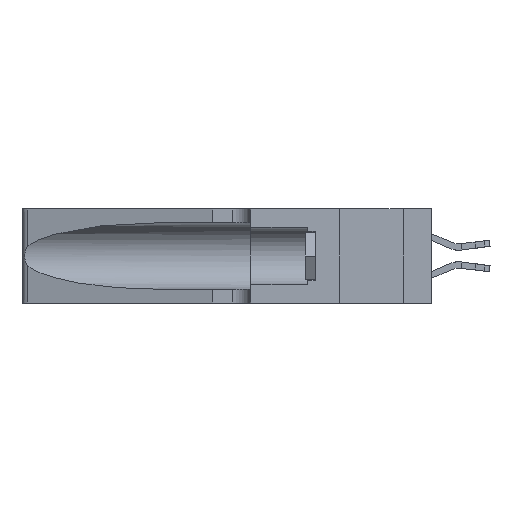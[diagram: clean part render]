
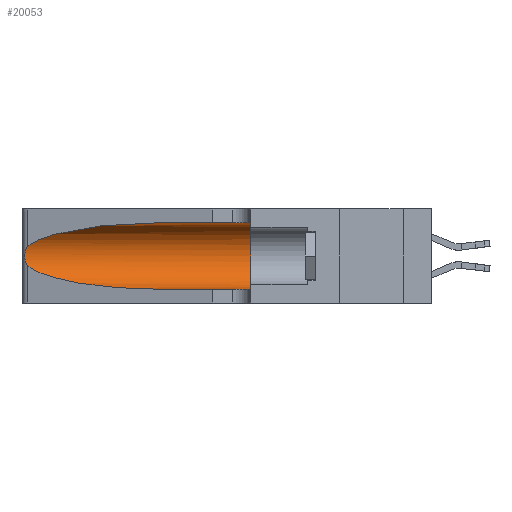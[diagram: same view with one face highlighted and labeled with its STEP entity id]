
A CAD part, left-side view. The second image highlights one B-rep face of the part: STEP entity #20053.
In plain terms, the highlighted cylindrical face has radius 3.308 mm (diameter 6.617 mm), a partial arc.
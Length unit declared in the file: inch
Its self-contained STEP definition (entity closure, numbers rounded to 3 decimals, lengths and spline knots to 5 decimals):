
#73 = B_SPLINE_CURVE_WITH_KNOTS ( 'NONE', 3,
 ( #13651, #1117, #9318, #3295, #23858, #24483, #26565, #3387, #9953, #1459, #24572, #22647, #10691, #15704 ),
 .UNSPECIFIED., .F., .F.,
 ( 4, 2, 2, 2, 2, 2, 4 ),
 ( 0., 0.00027, 0.00053, 0.00107, 0.0016, 0.00187, 0.00214 ),
 .UNSPECIFIED. ) ;
#98 = DIRECTION ( 'NONE',  ( 0., -1., 0. ) ) ;
#560 = ORIENTED_EDGE ( 'NONE', *, *, #17639, .T. ) ;
#666 = VERTEX_POINT ( 'NONE', #25088 ) ;
#972 = DIRECTION ( 'NONE',  ( 0., -1., 0. ) ) ;
#1107 = DIRECTION ( 'NONE',  ( 0., 0., 1. ) ) ;
#1117 = CARTESIAN_POINT ( 'NONE',  ( 0.25555, 1.22994, 0.2215 ) ) ;
#1459 = CARTESIAN_POINT ( 'NONE',  ( 0.25856, 1.23593, 0.16098 ) ) ;
#1947 = CARTESIAN_POINT ( 'NONE',  ( 0.2373, 1.15595, 0.08982 ) ) ;
#2285 = VERTEX_POINT ( 'NONE', #23830 ) ;
#2407 =( BOUNDED_CURVE ( )  B_SPLINE_CURVE ( 3, ( #6044, #1947, #22855, #18428 ),
 .UNSPECIFIED., .F., .F. ) 
 B_SPLINE_CURVE_WITH_KNOTS ( ( 4, 4 ),
 ( 3.44316, 4.71239 ),
 .UNSPECIFIED. ) 
 CURVE ( )  GEOMETRIC_REPRESENTATION_ITEM ( )  RATIONAL_B_SPLINE_CURVE ( ( 1., 0.87, 0.87, 1. ) ) 
 REPRESENTATION_ITEM ( '' )  );
#2459 = VECTOR ( 'NONE', #98, 39.37008 ) ;
#2837 = LINE ( 'NONE', #11319, #24513 ) ;
#3295 = CARTESIAN_POINT ( 'NONE',  ( 0.25787, 1.23484, 0.2124 ) ) ;
#3387 = CARTESIAN_POINT ( 'NONE',  ( 0.26075, 1.23896, 0.178 ) ) ;
#4401 =( BOUNDED_CURVE ( )  B_SPLINE_CURVE ( 3, ( #18512, #8134, #5947, #8233 ),
 .UNSPECIFIED., .F., .F. ) 
 B_SPLINE_CURVE_WITH_KNOTS ( ( 4, 4 ),
 ( 1.5708, 2.84003 ),
 .UNSPECIFIED. ) 
 CURVE ( )  GEOMETRIC_REPRESENTATION_ITEM ( )  RATIONAL_B_SPLINE_CURVE ( ( 1., 0.87, 0.87, 1. ) ) 
 REPRESENTATION_ITEM ( '' )  );
#4848 = CARTESIAN_POINT ( 'NONE',  ( 0.25487, 1.22718, 0.14631 ) ) ;
#5024 = EDGE_CURVE ( 'NONE', #666, #26345, #19876, .T. ) ;
#5606 = FACE_OUTER_BOUND ( 'NONE', #20737, .T. ) ;
#5947 = CARTESIAN_POINT ( 'NONE',  ( 0.2373, 1.15595, 0.28018 ) ) ;
#6044 = CARTESIAN_POINT ( 'NONE',  ( 0.25487, 1.22718, 0.14631 ) ) ;
#7119 = CARTESIAN_POINT ( 'NONE',  ( 0.1305, 0.35, 0.185 ) ) ;
#7221 = CARTESIAN_POINT ( 'NONE',  ( 0.1305, 0.72297, 0.31525 ) ) ;
#7569 = ORIENTED_EDGE ( 'NONE', *, *, #24463, .T. ) ;
#8015 = LINE ( 'NONE', #18783, #2459 ) ;
#8133 = DIRECTION ( 'NONE',  ( 0., 0., -1. ) ) ;
#8134 = CARTESIAN_POINT ( 'NONE',  ( 0.18966, 0.96281, 0.31525 ) ) ;
#8233 = CARTESIAN_POINT ( 'NONE',  ( 0.25487, 1.22718, 0.22369 ) ) ;
#8705 = ORIENTED_EDGE ( 'NONE', *, *, #5024, .F. ) ;
#9318 = CARTESIAN_POINT ( 'NONE',  ( 0.25639, 1.23184, 0.21858 ) ) ;
#9953 = CARTESIAN_POINT ( 'NONE',  ( 0.26017, 1.23833, 0.17102 ) ) ;
#10149 = CARTESIAN_POINT ( 'NONE',  ( 0.1305, 1.61858, 0.185 ) ) ;
#10691 = CARTESIAN_POINT ( 'NONE',  ( 0.25555, 1.22993, 0.14849 ) ) ;
#11019 = AXIS2_PLACEMENT_3D ( 'NONE', #7119, #13642, #1107 ) ;
#11319 = CARTESIAN_POINT ( 'NONE',  ( 0.1305, 1.61858, 0.31525 ) ) ;
#11947 = CARTESIAN_POINT ( 'NONE',  ( 0.1305, 0.35, 0.05475 ) ) ;
#12309 = DIRECTION ( 'NONE',  ( 0., -1., 0. ) ) ;
#12552 = VERTEX_POINT ( 'NONE', #7221 ) ;
#13642 = DIRECTION ( 'NONE',  ( 0., 1., 0. ) ) ;
#13651 = CARTESIAN_POINT ( 'NONE',  ( 0.25487, 1.22718, 0.22369 ) ) ;
#13914 = AXIS2_PLACEMENT_3D ( 'NONE', #10149, #12309, #8133 ) ;
#15390 = EDGE_CURVE ( 'NONE', #17275, #2285, #2407, .T. ) ;
#15704 = CARTESIAN_POINT ( 'NONE',  ( 0.25487, 1.22718, 0.14631 ) ) ;
#17275 = VERTEX_POINT ( 'NONE', #4848 ) ;
#17639 = EDGE_CURVE ( 'NONE', #12552, #23999, #4401, .T. ) ;
#18083 = CYLINDRICAL_SURFACE ( 'NONE', #13914, 0.13025 ) ;
#18428 = CARTESIAN_POINT ( 'NONE',  ( 0.1305, 0.72297, 0.05475 ) ) ;
#18512 = CARTESIAN_POINT ( 'NONE',  ( 0.1305, 0.72297, 0.31525 ) ) ;
#18783 = CARTESIAN_POINT ( 'NONE',  ( 0.1305, 1.61858, 0.05475 ) ) ;
#19058 = EDGE_CURVE ( 'NONE', #23999, #17275, #73, .T. ) ;
#19876 = CIRCLE ( 'NONE', #11019, 0.13025 ) ;
#20053 = ADVANCED_FACE ( 'NONE', ( #5606 ), #18083, .F. ) ;
#20737 = EDGE_LOOP ( 'NONE', ( #560, #23795, #23479, #7569, #8705, #27086 ) ) ;
#21829 = CARTESIAN_POINT ( 'NONE',  ( 0.25487, 1.22718, 0.22369 ) ) ;
#22647 = CARTESIAN_POINT ( 'NONE',  ( 0.25639, 1.23186, 0.15144 ) ) ;
#22855 = CARTESIAN_POINT ( 'NONE',  ( 0.18966, 0.96281, 0.05475 ) ) ;
#23373 = EDGE_CURVE ( 'NONE', #12552, #666, #2837, .T. ) ;
#23479 = ORIENTED_EDGE ( 'NONE', *, *, #15390, .T. ) ;
#23795 = ORIENTED_EDGE ( 'NONE', *, *, #19058, .T. ) ;
#23830 = CARTESIAN_POINT ( 'NONE',  ( 0.1305, 0.72297, 0.05475 ) ) ;
#23858 = CARTESIAN_POINT ( 'NONE',  ( 0.25854, 1.2359, 0.20912 ) ) ;
#23999 = VERTEX_POINT ( 'NONE', #21829 ) ;
#24463 = EDGE_CURVE ( 'NONE', #2285, #26345, #8015, .T. ) ;
#24483 = CARTESIAN_POINT ( 'NONE',  ( 0.26018, 1.23835, 0.19895 ) ) ;
#24513 = VECTOR ( 'NONE', #972, 39.37008 ) ;
#24572 = CARTESIAN_POINT ( 'NONE',  ( 0.25789, 1.23486, 0.15765 ) ) ;
#25088 = CARTESIAN_POINT ( 'NONE',  ( 0.1305, 0.35, 0.31525 ) ) ;
#26345 = VERTEX_POINT ( 'NONE', #11947 ) ;
#26565 = CARTESIAN_POINT ( 'NONE',  ( 0.26075, 1.23896, 0.19203 ) ) ;
#27086 = ORIENTED_EDGE ( 'NONE', *, *, #23373, .F. ) ;
